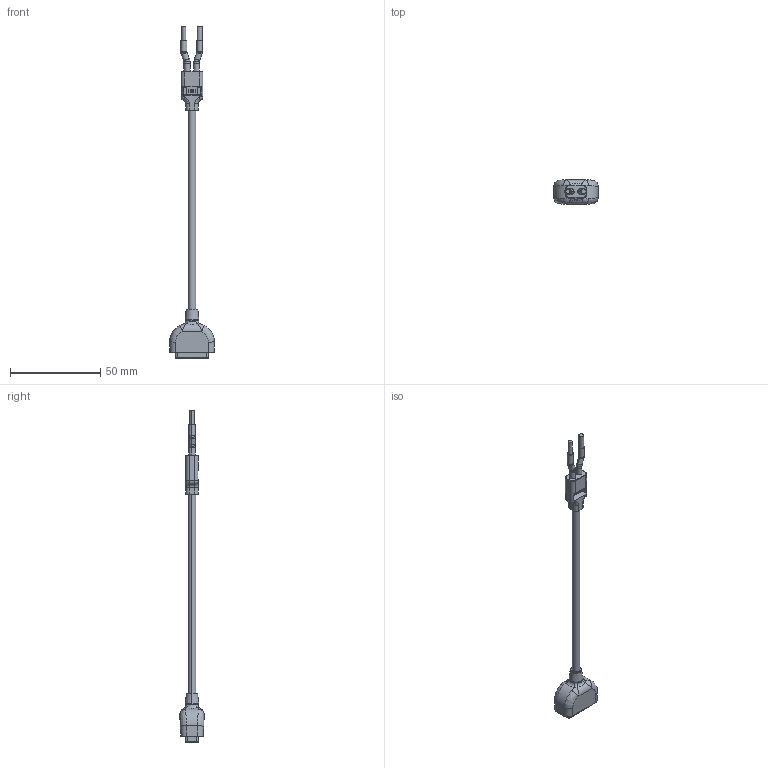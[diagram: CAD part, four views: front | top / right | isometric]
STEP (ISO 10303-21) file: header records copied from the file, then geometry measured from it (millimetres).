
FILE_DESCRIPTION (( 'STEP AP214' ), '1' );
FILE_NAME ('687K05510501138.STEP', '2023-05-05T19:29:55', ( '' ), ( '' ), 'SwSTEP 2.0', 'SolidWorks 2020', '' );
FILE_SCHEMA (( 'AUTOMOTIVE_DESIGN' ));
Length unit declared in the file: millimetre
Products named in the file (1): 687K05510501138
Bounding box: 24.7 x 13.55 x 184 mm (x, y, z)
Volume: 8174.7 mm3; surface area: 5035.9 mm2
Topology: 1 solids, 3 shells, 308 faces, 716 edges, 435 vertices
Faces by surface type: plane 105, cylinder 100, torus 47, bspline 46, cone 6, sphere 4
Entity records: 14458 total; most frequent: CARTESIAN_POINT 4824, DIRECTION 1432, ORIENTED_EDGE 1424, EDGE_CURVE 712, AXIS2_PLACEMENT_3D 551, VERTEX_POINT 435, EDGE_LOOP 337, LINE 330
